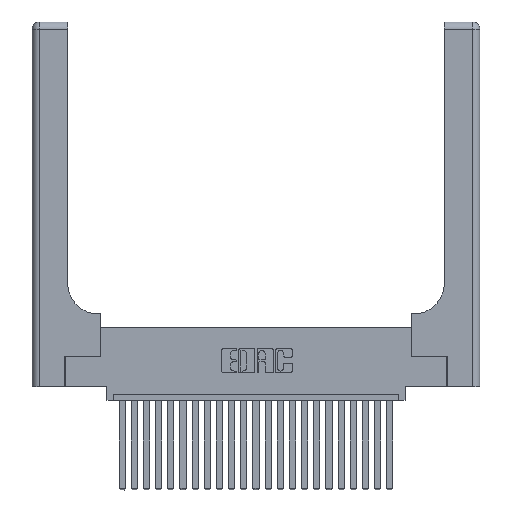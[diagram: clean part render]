
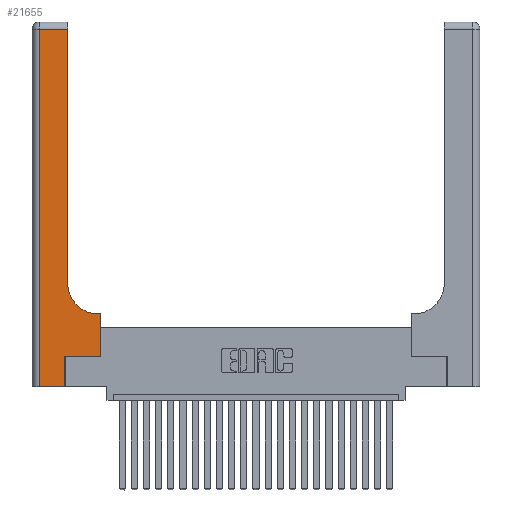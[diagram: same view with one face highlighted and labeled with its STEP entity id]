
A CAD part, top view. The second image highlights one B-rep face of the part: STEP entity #21655.
In plain terms, the highlighted planar face has unit normal (0, 0, 1).
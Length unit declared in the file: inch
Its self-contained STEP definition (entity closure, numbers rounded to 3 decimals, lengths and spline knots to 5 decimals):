
#358 = VECTOR ( 'NONE', #2274, 39.37008 ) ;
#828 = EDGE_CURVE ( 'NONE', #19399, #3798, #2980, .T. ) ;
#1752 = DIRECTION ( 'NONE',  ( 1., 0., 0. ) ) ;
#2206 = CARTESIAN_POINT ( 'NONE',  ( 0.269, 0.25, 0.37 ) ) ;
#2230 = LINE ( 'NONE', #20275, #15225 ) ;
#2274 = DIRECTION ( 'NONE',  ( 0., 1., 0. ) ) ;
#2980 = LINE ( 'NONE', #5023, #21074 ) ;
#3043 = VECTOR ( 'NONE', #24151, 39.37008 ) ;
#3213 = ORIENTED_EDGE ( 'NONE', *, *, #15834, .T. ) ;
#3295 = DIRECTION ( 'NONE',  ( -1., 0., 0. ) ) ;
#3300 = DIRECTION ( 'NONE',  ( -1., 0., 0. ) ) ;
#3502 = CARTESIAN_POINT ( 'NONE',  ( 0.269, 0., 0.37 ) ) ;
#3798 = VERTEX_POINT ( 'NONE', #19701 ) ;
#3863 = DIRECTION ( 'NONE',  ( 0., 1., 0. ) ) ;
#4144 = VECTOR ( 'NONE', #3300, 39.37008 ) ;
#4291 = CARTESIAN_POINT ( 'NONE',  ( 0.5415, 0.6, 0.37 ) ) ;
#5023 = CARTESIAN_POINT ( 'NONE',  ( 0.06, 3., 0.37 ) ) ;
#5060 = CARTESIAN_POINT ( 'NONE',  ( 0., 2.94, 0.37 ) ) ;
#5742 = CIRCLE ( 'NONE', #19042, 0.25 ) ;
#5849 = VERTEX_POINT ( 'NONE', #21202 ) ;
#6166 = ORIENTED_EDGE ( 'NONE', *, *, #13687, .T. ) ;
#6454 = CARTESIAN_POINT ( 'NONE',  ( 0., 0., 0.37 ) ) ;
#6746 = FACE_OUTER_BOUND ( 'NONE', #7707, .T. ) ;
#7201 = LINE ( 'NONE', #10966, #4144 ) ;
#7380 = LINE ( 'NONE', #21476, #358 ) ;
#7668 = CARTESIAN_POINT ( 'NONE',  ( 0., 3., 0.37 ) ) ;
#7707 = EDGE_LOOP ( 'NONE', ( #15824, #10798, #16569, #21625, #3213, #19930, #6166, #14271, #18795 ) ) ;
#8206 = CARTESIAN_POINT ( 'NONE',  ( 0.5585, 0.25, 0.37 ) ) ;
#8408 = LINE ( 'NONE', #5060, #16859 ) ;
#9073 = EDGE_CURVE ( 'NONE', #23358, #22132, #5742, .T. ) ;
#9105 = LINE ( 'NONE', #11379, #17839 ) ;
#9337 = AXIS2_PLACEMENT_3D ( 'NONE', #7668, #21320, #15639 ) ;
#9394 = LINE ( 'NONE', #12344, #3043 ) ;
#9477 = LINE ( 'NONE', #6454, #18548 ) ;
#10503 = DIRECTION ( 'NONE',  ( 0., -1., 0. ) ) ;
#10798 = ORIENTED_EDGE ( 'NONE', *, *, #11917, .T. ) ;
#10966 = CARTESIAN_POINT ( 'NONE',  ( 0.2915, 0.6, 0.37 ) ) ;
#11300 = CARTESIAN_POINT ( 'NONE',  ( 0.5415, 0.85, 0.37 ) ) ;
#11379 = CARTESIAN_POINT ( 'NONE',  ( 0.2915, 3., 0.37 ) ) ;
#11763 = PLANE ( 'NONE',  #9337 ) ;
#11917 = EDGE_CURVE ( 'NONE', #5849, #19399, #8408, .T. ) ;
#12344 = CARTESIAN_POINT ( 'NONE',  ( 0.269, 0.25, 0.37 ) ) ;
#13231 = DIRECTION ( 'NONE',  ( 0., 0., -1. ) ) ;
#13687 = EDGE_CURVE ( 'NONE', #13944, #15147, #2230, .T. ) ;
#13884 = DIRECTION ( 'NONE',  ( 1., 0., 0. ) ) ;
#13944 = VERTEX_POINT ( 'NONE', #8206 ) ;
#14039 = CARTESIAN_POINT ( 'NONE',  ( 0.2915, 0.85, 0.37 ) ) ;
#14192 = DIRECTION ( 'NONE',  ( 0., 1., 0. ) ) ;
#14271 = ORIENTED_EDGE ( 'NONE', *, *, #19659, .T. ) ;
#15147 = VERTEX_POINT ( 'NONE', #20638 ) ;
#15225 = VECTOR ( 'NONE', #14192, 39.37008 ) ;
#15639 = DIRECTION ( 'NONE',  ( -1., 0., 0. ) ) ;
#15824 = ORIENTED_EDGE ( 'NONE', *, *, #18136, .T. ) ;
#15834 = EDGE_CURVE ( 'NONE', #20869, #16983, #7380, .T. ) ;
#16569 = ORIENTED_EDGE ( 'NONE', *, *, #828, .T. ) ;
#16859 = VECTOR ( 'NONE', #3295, 39.37008 ) ;
#16983 = VERTEX_POINT ( 'NONE', #2206 ) ;
#17839 = VECTOR ( 'NONE', #3863, 39.37008 ) ;
#18136 = EDGE_CURVE ( 'NONE', #22132, #5849, #9105, .T. ) ;
#18548 = VECTOR ( 'NONE', #13884, 39.37008 ) ;
#18795 = ORIENTED_EDGE ( 'NONE', *, *, #9073, .T. ) ;
#19042 = AXIS2_PLACEMENT_3D ( 'NONE', #11300, #13231, #1752 ) ;
#19399 = VERTEX_POINT ( 'NONE', #19819 ) ;
#19659 = EDGE_CURVE ( 'NONE', #15147, #23358, #7201, .T. ) ;
#19701 = CARTESIAN_POINT ( 'NONE',  ( 0.06, 0., 0.37 ) ) ;
#19819 = CARTESIAN_POINT ( 'NONE',  ( 0.06, 2.94, 0.37 ) ) ;
#19930 = ORIENTED_EDGE ( 'NONE', *, *, #24190, .T. ) ;
#20275 = CARTESIAN_POINT ( 'NONE',  ( 0.5585, 0.25, 0.37 ) ) ;
#20638 = CARTESIAN_POINT ( 'NONE',  ( 0.5585, 0.6, 0.37 ) ) ;
#20869 = VERTEX_POINT ( 'NONE', #3502 ) ;
#21074 = VECTOR ( 'NONE', #10503, 39.37008 ) ;
#21202 = CARTESIAN_POINT ( 'NONE',  ( 0.2915, 2.94, 0.37 ) ) ;
#21320 = DIRECTION ( 'NONE',  ( 0., 0., -1. ) ) ;
#21476 = CARTESIAN_POINT ( 'NONE',  ( 0.269, 0., 0.37 ) ) ;
#21625 = ORIENTED_EDGE ( 'NONE', *, *, #21813, .T. ) ;
#21655 = ADVANCED_FACE ( 'NONE', ( #6746 ), #11763, .F. ) ;
#21813 = EDGE_CURVE ( 'NONE', #3798, #20869, #9477, .T. ) ;
#22132 = VERTEX_POINT ( 'NONE', #14039 ) ;
#23358 = VERTEX_POINT ( 'NONE', #4291 ) ;
#24151 = DIRECTION ( 'NONE',  ( 1., 0., 0. ) ) ;
#24190 = EDGE_CURVE ( 'NONE', #16983, #13944, #9394, .T. ) ;
